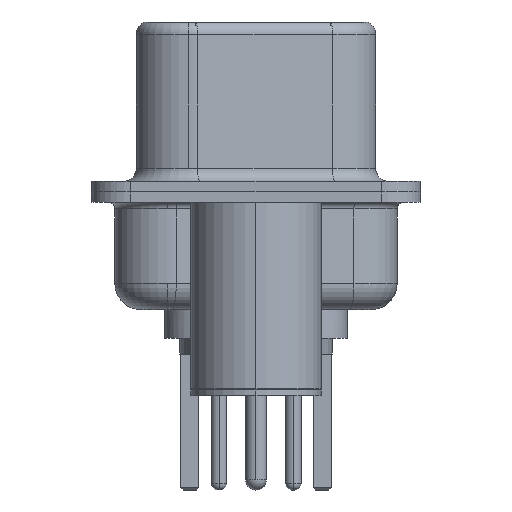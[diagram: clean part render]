
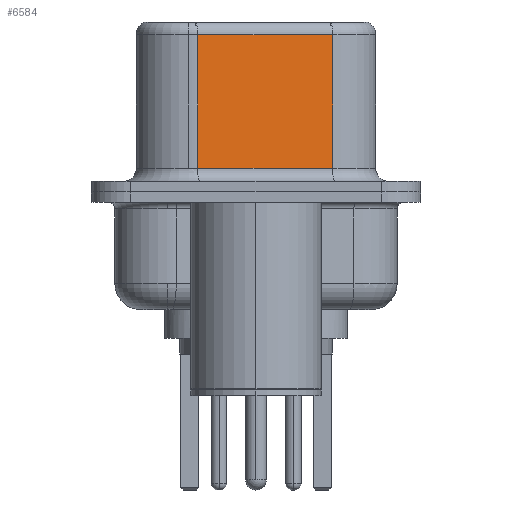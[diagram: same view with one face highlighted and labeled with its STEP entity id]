
A CAD part, left-side view. The second image highlights one B-rep face of the part: STEP entity #6584.
In plain terms, the highlighted planar face has unit normal (-0.985, -0.174, 0).
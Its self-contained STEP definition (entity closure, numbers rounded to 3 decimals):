
#426 = VECTOR ( 'NONE', #12020, 1000. ) ;
#967 = CARTESIAN_POINT ( 'NONE',  ( 3.67, 2.233, 0.9 ) ) ;
#986 = CARTESIAN_POINT ( 'NONE',  ( 4.58, -2.927, 6.02 ) ) ;
#1036 = DIRECTION ( 'NONE',  ( -0.174, 0.985, 0. ) ) ;
#2291 = LINE ( 'NONE', #986, #20470 ) ;
#2340 = VERTEX_POINT ( 'NONE', #7871 ) ;
#2985 = CARTESIAN_POINT ( 'NONE',  ( 4.58, -2.927, 0.9 ) ) ;
#3271 = DIRECTION ( 'NONE',  ( -0.174, 0.985, 0. ) ) ;
#4062 = LINE ( 'NONE', #6907, #8705 ) ;
#4127 = VERTEX_POINT ( 'NONE', #7175 ) ;
#4326 = CARTESIAN_POINT ( 'NONE',  ( 3.67, 2.233, 6.52 ) ) ;
#4445 = ORIENTED_EDGE ( 'NONE', *, *, #20979, .T. ) ;
#6536 = CARTESIAN_POINT ( 'NONE',  ( 4.58, -2.927, 6.02 ) ) ;
#6584 = ADVANCED_FACE ( 'NONE', ( #16176 ), #14590, .F. ) ;
#6907 = CARTESIAN_POINT ( 'NONE',  ( 4.58, -2.927, 6.52 ) ) ;
#7175 = CARTESIAN_POINT ( 'NONE',  ( 3.67, 2.233, 6.02 ) ) ;
#7871 = CARTESIAN_POINT ( 'NONE',  ( 4.58, -2.927, 0.9 ) ) ;
#8658 = EDGE_CURVE ( 'NONE', #16389, #2340, #19307, .T. ) ;
#8705 = VECTOR ( 'NONE', #13755, 1000. ) ;
#8984 = VECTOR ( 'NONE', #22546, 1000. ) ;
#12020 = DIRECTION ( 'NONE',  ( 0.174, -0.985, 0. ) ) ;
#13755 = DIRECTION ( 'NONE',  ( 0., 0., -1. ) ) ;
#14513 = ORIENTED_EDGE ( 'NONE', *, *, #8658, .T. ) ;
#14590 = PLANE ( 'NONE',  #29249 ) ;
#14676 = DIRECTION ( 'NONE',  ( 0.985, 0.174, 0. ) ) ;
#15036 = LINE ( 'NONE', #4326, #8984 ) ;
#16176 = FACE_OUTER_BOUND ( 'NONE', #17873, .T. ) ;
#16389 = VERTEX_POINT ( 'NONE', #967 ) ;
#17873 = EDGE_LOOP ( 'NONE', ( #29450, #24083, #4445, #14513 ) ) ;
#19307 = LINE ( 'NONE', #2985, #426 ) ;
#20470 = VECTOR ( 'NONE', #3271, 1000. ) ;
#20979 = EDGE_CURVE ( 'NONE', #4127, #16389, #15036, .T. ) ;
#22546 = DIRECTION ( 'NONE',  ( 0., 0., -1. ) ) ;
#22977 = EDGE_CURVE ( 'NONE', #25224, #2340, #4062, .T. ) ;
#23294 = EDGE_CURVE ( 'NONE', #25224, #4127, #2291, .T. ) ;
#23746 = CARTESIAN_POINT ( 'NONE',  ( 4.58, -2.927, 6.52 ) ) ;
#24083 = ORIENTED_EDGE ( 'NONE', *, *, #23294, .T. ) ;
#25224 = VERTEX_POINT ( 'NONE', #6536 ) ;
#29249 = AXIS2_PLACEMENT_3D ( 'NONE', #23746, #14676, #1036 ) ;
#29450 = ORIENTED_EDGE ( 'NONE', *, *, #22977, .F. ) ;
